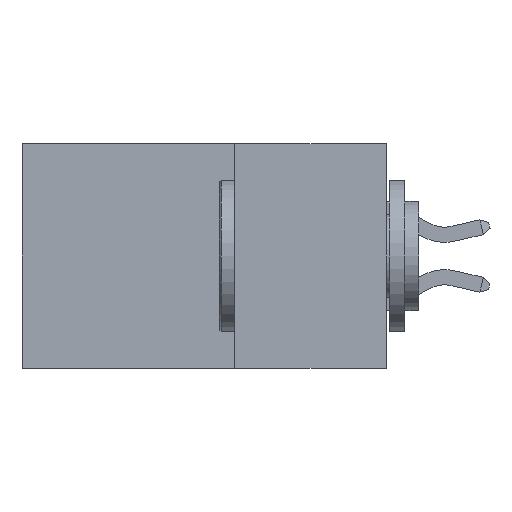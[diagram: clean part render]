
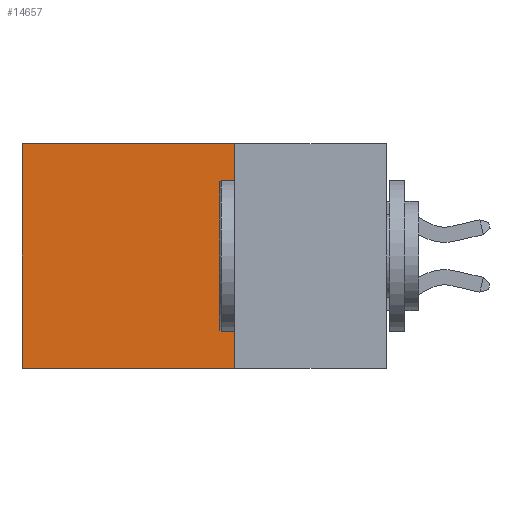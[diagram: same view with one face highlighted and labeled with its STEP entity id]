
A CAD part, left-side view. The second image highlights one B-rep face of the part: STEP entity #14657.
In plain terms, the highlighted planar face has unit normal (-1, 0, 0).
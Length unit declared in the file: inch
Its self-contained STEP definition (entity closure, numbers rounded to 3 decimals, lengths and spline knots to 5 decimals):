
#473 = CARTESIAN_POINT ( 'NONE',  ( 0.298, 0.25, -0.37 ) ) ;
#1301 = DIRECTION ( 'NONE',  ( 0., 0., -1. ) ) ;
#2597 = FACE_OUTER_BOUND ( 'NONE', #13437, .T. ) ;
#4507 = CARTESIAN_POINT ( 'NONE',  ( 0.298, 0.6, 0. ) ) ;
#5493 = VECTOR ( 'NONE', #18834, 39.37008 ) ;
#6244 = VERTEX_POINT ( 'NONE', #4507 ) ;
#6559 = EDGE_CURVE ( 'NONE', #6244, #11250, #23834, .T. ) ;
#6869 = EDGE_CURVE ( 'NONE', #22815, #11250, #11000, .T. ) ;
#7489 = VECTOR ( 'NONE', #11165, 39.37008 ) ;
#7581 = DIRECTION ( 'NONE',  ( 0., 1., 0. ) ) ;
#7798 = VECTOR ( 'NONE', #23780, 39.37008 ) ;
#8670 = CARTESIAN_POINT ( 'NONE',  ( 0.298, 0.25, -0.37 ) ) ;
#9099 = CARTESIAN_POINT ( 'NONE',  ( 0.298, 0.25, 0. ) ) ;
#9574 = EDGE_CURVE ( 'NONE', #18912, #22815, #18288, .T. ) ;
#10579 = CARTESIAN_POINT ( 'NONE',  ( 0.298, 0.25, 0. ) ) ;
#11000 = LINE ( 'NONE', #8670, #5493 ) ;
#11165 = DIRECTION ( 'NONE',  ( 0., 0., -1. ) ) ;
#11250 = VERTEX_POINT ( 'NONE', #20249 ) ;
#11806 = ORIENTED_EDGE ( 'NONE', *, *, #6869, .F. ) ;
#13077 = AXIS2_PLACEMENT_3D ( 'NONE', #25671, #13746, #1301 ) ;
#13437 = EDGE_LOOP ( 'NONE', ( #18703, #11806, #15492, #18036 ) ) ;
#13746 = DIRECTION ( 'NONE',  ( 1., 0., 0. ) ) ;
#13828 = CARTESIAN_POINT ( 'NONE',  ( 0.298, 0.6, 0. ) ) ;
#14657 = ADVANCED_FACE ( 'NONE', ( #2597 ), #23698, .F. ) ;
#15492 = ORIENTED_EDGE ( 'NONE', *, *, #9574, .F. ) ;
#16063 = LINE ( 'NONE', #19698, #16704 ) ;
#16704 = VECTOR ( 'NONE', #7581, 39.37008 ) ;
#17309 = EDGE_CURVE ( 'NONE', #18912, #6244, #16063, .T. ) ;
#18036 = ORIENTED_EDGE ( 'NONE', *, *, #17309, .T. ) ;
#18288 = LINE ( 'NONE', #9099, #7489 ) ;
#18703 = ORIENTED_EDGE ( 'NONE', *, *, #6559, .T. ) ;
#18834 = DIRECTION ( 'NONE',  ( 0., 1., 0. ) ) ;
#18912 = VERTEX_POINT ( 'NONE', #10579 ) ;
#19698 = CARTESIAN_POINT ( 'NONE',  ( 0.298, 0.25, 0. ) ) ;
#20249 = CARTESIAN_POINT ( 'NONE',  ( 0.298, 0.6, -0.37 ) ) ;
#22815 = VERTEX_POINT ( 'NONE', #473 ) ;
#23698 = PLANE ( 'NONE',  #13077 ) ;
#23780 = DIRECTION ( 'NONE',  ( 0., 0., -1. ) ) ;
#23834 = LINE ( 'NONE', #13828, #7798 ) ;
#25671 = CARTESIAN_POINT ( 'NONE',  ( 0.298, 0.25, 0. ) ) ;
